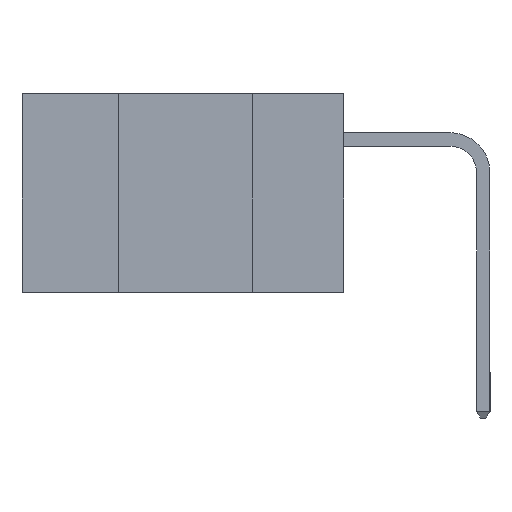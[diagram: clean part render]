
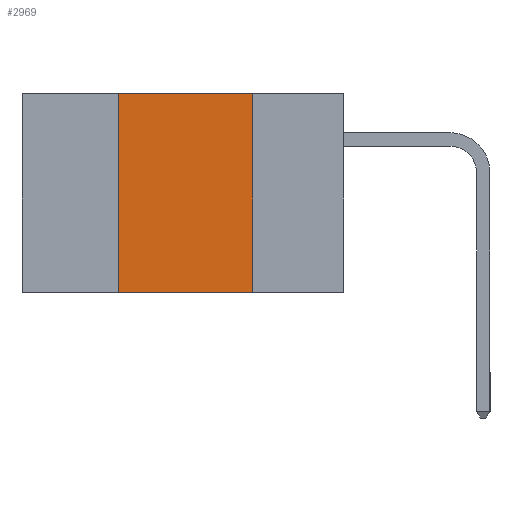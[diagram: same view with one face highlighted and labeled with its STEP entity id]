
A CAD part, left-side view. The second image highlights one B-rep face of the part: STEP entity #2969.
In plain terms, the highlighted planar face has unit normal (-1, 0, 0).
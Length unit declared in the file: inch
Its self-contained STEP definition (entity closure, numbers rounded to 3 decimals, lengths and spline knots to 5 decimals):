
#754 = CARTESIAN_POINT ( 'NONE',  ( 0., 0.6, 0. ) ) ;
#848 = CARTESIAN_POINT ( 'NONE',  ( 0., 0.42, -0.37 ) ) ;
#1760 = CARTESIAN_POINT ( 'NONE',  ( 0., 0.42, 0. ) ) ;
#2449 = CARTESIAN_POINT ( 'NONE',  ( 0., 0.17, -0.37 ) ) ;
#2587 = VERTEX_POINT ( 'NONE', #5678 ) ;
#2778 = AXIS2_PLACEMENT_3D ( 'NONE', #11307, #3192, #8307 ) ;
#2969 = ADVANCED_FACE ( 'NONE', ( #8203 ), #16221, .F. ) ;
#3192 = DIRECTION ( 'NONE',  ( 1., 0., 0. ) ) ;
#5157 = EDGE_LOOP ( 'NONE', ( #17153, #20981, #10363, #7271 ) ) ;
#5678 = CARTESIAN_POINT ( 'NONE',  ( 0., 0.17, 0. ) ) ;
#5803 = VECTOR ( 'NONE', #6510, 39.37008 ) ;
#6026 = EDGE_CURVE ( 'NONE', #13498, #8419, #15915, .T. ) ;
#6510 = DIRECTION ( 'NONE',  ( 0., -1., 0. ) ) ;
#7266 = DIRECTION ( 'NONE',  ( 0., -1., 0. ) ) ;
#7271 = ORIENTED_EDGE ( 'NONE', *, *, #14896, .T. ) ;
#8108 = CARTESIAN_POINT ( 'NONE',  ( 0., 0.6, -0.37 ) ) ;
#8203 = FACE_OUTER_BOUND ( 'NONE', #5157, .T. ) ;
#8307 = DIRECTION ( 'NONE',  ( 0., 0., -1. ) ) ;
#8419 = VERTEX_POINT ( 'NONE', #1760 ) ;
#9510 = LINE ( 'NONE', #8108, #5803 ) ;
#10363 = ORIENTED_EDGE ( 'NONE', *, *, #6026, .F. ) ;
#11010 = LINE ( 'NONE', #754, #19872 ) ;
#11212 = VECTOR ( 'NONE', #14228, 39.37008 ) ;
#11307 = CARTESIAN_POINT ( 'NONE',  ( 0., 0.6, 0. ) ) ;
#12134 = VERTEX_POINT ( 'NONE', #20217 ) ;
#12508 = CARTESIAN_POINT ( 'NONE',  ( 0., 0.42, -0.37 ) ) ;
#12839 = EDGE_CURVE ( 'NONE', #8419, #2587, #11010, .T. ) ;
#13498 = VERTEX_POINT ( 'NONE', #848 ) ;
#14228 = DIRECTION ( 'NONE',  ( 0., 0., 1. ) ) ;
#14896 = EDGE_CURVE ( 'NONE', #13498, #12134, #9510, .T. ) ;
#15487 = DIRECTION ( 'NONE',  ( 0., 0., -1. ) ) ;
#15915 = LINE ( 'NONE', #12508, #11212 ) ;
#15964 = EDGE_CURVE ( 'NONE', #2587, #12134, #18689, .T. ) ;
#16221 = PLANE ( 'NONE',  #2778 ) ;
#17153 = ORIENTED_EDGE ( 'NONE', *, *, #15964, .F. ) ;
#18689 = LINE ( 'NONE', #2449, #19120 ) ;
#19120 = VECTOR ( 'NONE', #15487, 39.37008 ) ;
#19872 = VECTOR ( 'NONE', #7266, 39.37008 ) ;
#20217 = CARTESIAN_POINT ( 'NONE',  ( 0., 0.17, -0.37 ) ) ;
#20981 = ORIENTED_EDGE ( 'NONE', *, *, #12839, .F. ) ;
